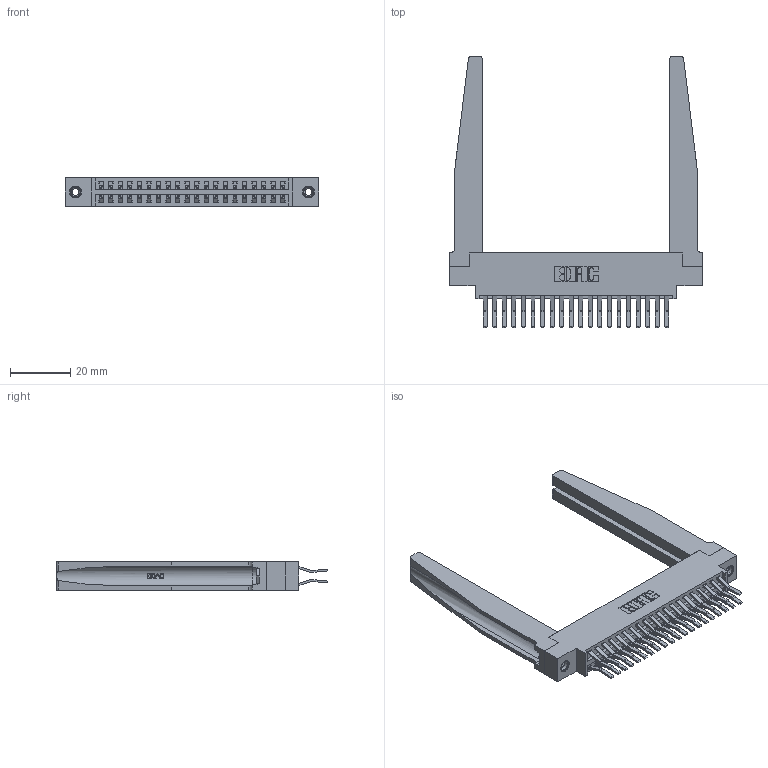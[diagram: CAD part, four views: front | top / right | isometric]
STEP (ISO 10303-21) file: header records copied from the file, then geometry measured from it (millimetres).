
FILE_DESCRIPTION (( 'STEP AP203' ), '1' );
FILE_NAME ('346-040-560-878.STEP', '2022-05-20T03:21:15', ( '' ), ( '' ), 'SwSTEP 2.0', 'SolidWorks 2020', '' );
FILE_SCHEMA (( 'CONFIG_CONTROL_DESIGN' ));
Length unit declared in the file: inch
Products named in the file (5): 345-292-001_560 Tail; 346-220-078_345-220-078; 345-250-001_345-250-001-102; 346 Part_0.170 Offset - 0.156 Dia-TH; 346-040-560-878
Assembly tree (45 placements, depth 2):
  346-040-560-878
    346 Part_0.170 Offset - 0.156 Dia-TH
    345-292-001_560 Tail  x40
    346-220-078_345-220-078  x2
    345-250-001_345-250-001-102  x2
Bounding box: 84.07 x 90.05 x 9.4 mm (x, y, z)
Volume: 15025.7 mm3; surface area: 18262.6 mm2
Topology: 45 solids, 45 shells, 2534 faces, 7425 edges, 4886 vertices
Faces by surface type: plane 1636, cylinder 846, bspline 36, cone 12, torus 4
Entity records: 21398 total; most frequent: CARTESIAN_POINT 4501, ORIENTED_EDGE 3322, DIRECTION 3007, EDGE_CURVE 1661, LINE 1351, VECTOR 1351, VERTEX_POINT 1100, AXIS2_PLACEMENT_3D 828
